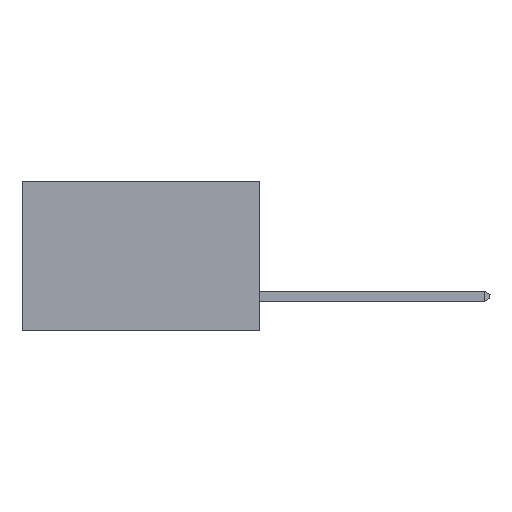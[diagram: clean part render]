
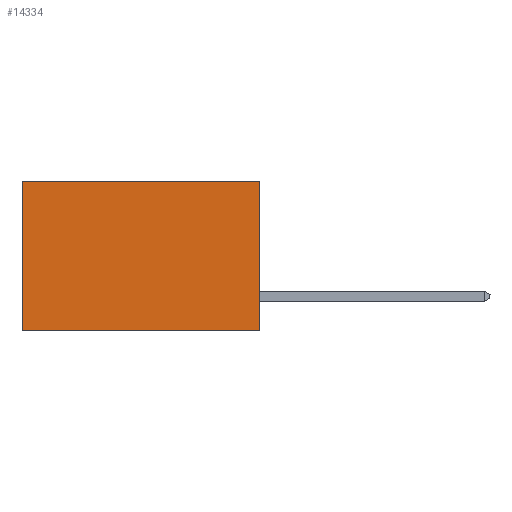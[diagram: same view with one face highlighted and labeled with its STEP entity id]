
A CAD part, left-side view. The second image highlights one B-rep face of the part: STEP entity #14334.
In plain terms, the highlighted planar face has unit normal (-1, 0, 0).
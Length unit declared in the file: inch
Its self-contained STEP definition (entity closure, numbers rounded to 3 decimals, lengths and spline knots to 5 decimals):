
#51 = CARTESIAN_POINT ( 'NONE',  ( 0.277, 0., 0. ) ) ;
#401 = FACE_OUTER_BOUND ( 'NONE', #2367, .T. ) ;
#998 = VERTEX_POINT ( 'NONE', #16586 ) ;
#2367 = EDGE_LOOP ( 'NONE', ( #2775, #7323, #7851, #12314 ) ) ;
#2775 = ORIENTED_EDGE ( 'NONE', *, *, #7738, .T. ) ;
#3305 = VERTEX_POINT ( 'NONE', #6248 ) ;
#3436 = CARTESIAN_POINT ( 'NONE',  ( 0.277, 0., -0.37 ) ) ;
#3967 = CARTESIAN_POINT ( 'NONE',  ( 0.277, 0., -0.37 ) ) ;
#4544 = CARTESIAN_POINT ( 'NONE',  ( 0.277, 0., -0.37 ) ) ;
#4618 = DIRECTION ( 'NONE',  ( 0., 1., 0. ) ) ;
#4889 = VECTOR ( 'NONE', #14856, 39.37008 ) ;
#5787 = PLANE ( 'NONE',  #15444 ) ;
#6212 = VECTOR ( 'NONE', #12078, 39.37008 ) ;
#6248 = CARTESIAN_POINT ( 'NONE',  ( 0.277, 0.59, -0.37 ) ) ;
#6560 = VERTEX_POINT ( 'NONE', #51 ) ;
#7323 = ORIENTED_EDGE ( 'NONE', *, *, #20154, .F. ) ;
#7691 = LINE ( 'NONE', #3436, #11611 ) ;
#7738 = EDGE_CURVE ( 'NONE', #998, #3305, #15136, .T. ) ;
#7851 = ORIENTED_EDGE ( 'NONE', *, *, #17975, .F. ) ;
#8976 = VERTEX_POINT ( 'NONE', #3967 ) ;
#9051 = LINE ( 'NONE', #4544, #12448 ) ;
#9206 = DIRECTION ( 'NONE',  ( 0., 0., -1. ) ) ;
#9829 = CARTESIAN_POINT ( 'NONE',  ( 0.277, 0., 0. ) ) ;
#10478 = LINE ( 'NONE', #9829, #4889 ) ;
#11611 = VECTOR ( 'NONE', #16863, 39.37008 ) ;
#12078 = DIRECTION ( 'NONE',  ( 0., 0., -1. ) ) ;
#12157 = CARTESIAN_POINT ( 'NONE',  ( 0.277, 0.59, -0.37 ) ) ;
#12314 = ORIENTED_EDGE ( 'NONE', *, *, #13185, .T. ) ;
#12448 = VECTOR ( 'NONE', #4618, 39.37008 ) ;
#13185 = EDGE_CURVE ( 'NONE', #6560, #998, #10478, .T. ) ;
#14334 = ADVANCED_FACE ( 'NONE', ( #401 ), #5787, .F. ) ;
#14856 = DIRECTION ( 'NONE',  ( 0., 1., 0. ) ) ;
#15136 = LINE ( 'NONE', #12157, #6212 ) ;
#15444 = AXIS2_PLACEMENT_3D ( 'NONE', #17455, #19041, #9206 ) ;
#16586 = CARTESIAN_POINT ( 'NONE',  ( 0.277, 0.59, 0. ) ) ;
#16863 = DIRECTION ( 'NONE',  ( 0., 0., -1. ) ) ;
#17455 = CARTESIAN_POINT ( 'NONE',  ( 0.277, 0., -0.37 ) ) ;
#17975 = EDGE_CURVE ( 'NONE', #6560, #8976, #7691, .T. ) ;
#19041 = DIRECTION ( 'NONE',  ( 1., 0., 0. ) ) ;
#20154 = EDGE_CURVE ( 'NONE', #8976, #3305, #9051, .T. ) ;
